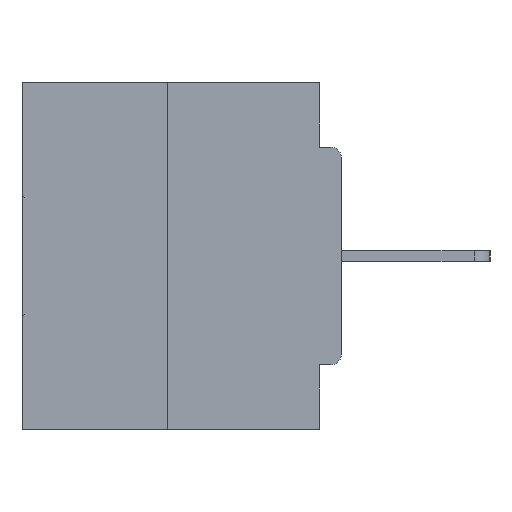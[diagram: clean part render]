
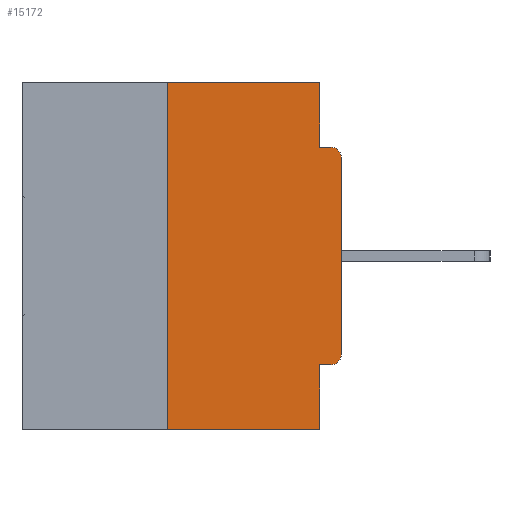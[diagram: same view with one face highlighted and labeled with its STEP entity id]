
A CAD part, left-side view. The second image highlights one B-rep face of the part: STEP entity #15172.
In plain terms, the highlighted planar face has unit normal (-1, 0, 0).
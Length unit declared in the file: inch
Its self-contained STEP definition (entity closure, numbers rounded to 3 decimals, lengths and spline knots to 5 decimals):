
#285 = ORIENTED_EDGE ( 'NONE', *, *, #29070, .F. ) ;
#410 = CARTESIAN_POINT ( 'NONE',  ( 0., 0., -0.1085 ) ) ;
#688 = CARTESIAN_POINT ( 'NONE',  ( 0., 0.25, -0.5 ) ) ;
#1033 = EDGE_CURVE ( 'NONE', #34294, #27503, #32344, .T. ) ;
#1077 = ORIENTED_EDGE ( 'NONE', *, *, #14385, .F. ) ;
#1330 = DIRECTION ( 'NONE',  ( 0., 0., -1. ) ) ;
#1719 = EDGE_CURVE ( 'NONE', #29266, #22250, #33570, .T. ) ;
#1813 = FACE_OUTER_BOUND ( 'NONE', #9121, .T. ) ;
#2770 = CARTESIAN_POINT ( 'NONE',  ( 0., 0.25, 0. ) ) ;
#3342 = DIRECTION ( 'NONE',  ( 0., 1., 0. ) ) ;
#4449 = AXIS2_PLACEMENT_3D ( 'NONE', #12134, #6806, #1330 ) ;
#4674 = DIRECTION ( 'NONE',  ( 0., -1., 0. ) ) ;
#5572 = VECTOR ( 'NONE', #19387, 39.37008 ) ;
#6806 = DIRECTION ( 'NONE',  ( -1., 0., 0. ) ) ;
#7591 = ORIENTED_EDGE ( 'NONE', *, *, #1033, .T. ) ;
#7671 = CARTESIAN_POINT ( 'NONE',  ( 0., 0.46, 0. ) ) ;
#7896 = CARTESIAN_POINT ( 'NONE',  ( 0., 0.015, -0.0935 ) ) ;
#8212 = LINE ( 'NONE', #17017, #31255 ) ;
#9121 = EDGE_LOOP ( 'NONE', ( #16696, #1077, #13691, #285, #24220, #7591, #22147, #12016, #12784, #18666 ) ) ;
#9130 = CARTESIAN_POINT ( 'NONE',  ( 0., 0.46, 0. ) ) ;
#9494 = LINE ( 'NONE', #31753, #15277 ) ;
#9628 = CARTESIAN_POINT ( 'NONE',  ( 0., 0.031, -0.5 ) ) ;
#9995 = EDGE_CURVE ( 'NONE', #34294, #20419, #28713, .T. ) ;
#10006 = VECTOR ( 'NONE', #3342, 39.37008 ) ;
#10246 = VERTEX_POINT ( 'NONE', #2770 ) ;
#10512 = CARTESIAN_POINT ( 'NONE',  ( 0., 0.031, -0.0935 ) ) ;
#10579 = CARTESIAN_POINT ( 'NONE',  ( 0., 0.031, 0. ) ) ;
#11364 = VERTEX_POINT ( 'NONE', #9628 ) ;
#11960 = VECTOR ( 'NONE', #4674, 39.37008 ) ;
#12016 = ORIENTED_EDGE ( 'NONE', *, *, #32471, .T. ) ;
#12068 = CARTESIAN_POINT ( 'NONE',  ( 0., 0.015, -0.3915 ) ) ;
#12134 = CARTESIAN_POINT ( 'NONE',  ( 0., 0.015, -0.1085 ) ) ;
#12256 = LINE ( 'NONE', #34728, #26589 ) ;
#12784 = ORIENTED_EDGE ( 'NONE', *, *, #13802, .F. ) ;
#13243 = LINE ( 'NONE', #35322, #24925 ) ;
#13640 = LINE ( 'NONE', #22123, #14757 ) ;
#13691 = ORIENTED_EDGE ( 'NONE', *, *, #24667, .T. ) ;
#13802 = EDGE_CURVE ( 'NONE', #22250, #20015, #12256, .T. ) ;
#13872 = CARTESIAN_POINT ( 'NONE',  ( 0., 0.031, 0. ) ) ;
#14203 = AXIS2_PLACEMENT_3D ( 'NONE', #7671, #15938, #15387 ) ;
#14385 = EDGE_CURVE ( 'NONE', #26643, #10246, #13640, .T. ) ;
#14757 = VECTOR ( 'NONE', #24898, 39.37008 ) ;
#15002 = DIRECTION ( 'NONE',  ( 0., -1., 0. ) ) ;
#15172 = ADVANCED_FACE ( 'NONE', ( #1813 ), #15579, .F. ) ;
#15277 = VECTOR ( 'NONE', #15002, 39.37008 ) ;
#15280 = EDGE_CURVE ( 'NONE', #27503, #33959, #8212, .T. ) ;
#15387 = DIRECTION ( 'NONE',  ( 0., 0., -1. ) ) ;
#15579 = PLANE ( 'NONE',  #14203 ) ;
#15938 = DIRECTION ( 'NONE',  ( 1., 0., 0. ) ) ;
#16317 = DIRECTION ( 'NONE',  ( 0., 0., 1. ) ) ;
#16696 = ORIENTED_EDGE ( 'NONE', *, *, #16737, .F. ) ;
#16737 = EDGE_CURVE ( 'NONE', #10246, #29266, #34343, .T. ) ;
#17017 = CARTESIAN_POINT ( 'NONE',  ( 0., 0., 0. ) ) ;
#17055 = CARTESIAN_POINT ( 'NONE',  ( 0., 0.015, -0.4065 ) ) ;
#17063 = CARTESIAN_POINT ( 'NONE',  ( 0., 0., -0.3915 ) ) ;
#18666 = ORIENTED_EDGE ( 'NONE', *, *, #1719, .F. ) ;
#19387 = DIRECTION ( 'NONE',  ( 0., 0., -1. ) ) ;
#20015 = VERTEX_POINT ( 'NONE', #7896 ) ;
#20419 = VERTEX_POINT ( 'NONE', #30483 ) ;
#22123 = CARTESIAN_POINT ( 'NONE',  ( 0., 0.25, 0. ) ) ;
#22147 = ORIENTED_EDGE ( 'NONE', *, *, #15280, .T. ) ;
#22250 = VERTEX_POINT ( 'NONE', #10512 ) ;
#23317 = DIRECTION ( 'NONE',  ( -1., 0., 0. ) ) ;
#23332 = DIRECTION ( 'NONE',  ( 0., -1., 0. ) ) ;
#24109 = DIRECTION ( 'NONE',  ( 0., 0., -1. ) ) ;
#24220 = ORIENTED_EDGE ( 'NONE', *, *, #9995, .F. ) ;
#24230 = DIRECTION ( 'NONE',  ( 0., 0., -1. ) ) ;
#24667 = EDGE_CURVE ( 'NONE', #26643, #11364, #9494, .T. ) ;
#24898 = DIRECTION ( 'NONE',  ( 0., 0., 1. ) ) ;
#24925 = VECTOR ( 'NONE', #24109, 39.37008 ) ;
#26589 = VECTOR ( 'NONE', #23332, 39.37008 ) ;
#26643 = VERTEX_POINT ( 'NONE', #688 ) ;
#27503 = VERTEX_POINT ( 'NONE', #17063 ) ;
#28713 = LINE ( 'NONE', #31833, #10006 ) ;
#29070 = EDGE_CURVE ( 'NONE', #20419, #11364, #13243, .T. ) ;
#29266 = VERTEX_POINT ( 'NONE', #10579 ) ;
#30483 = CARTESIAN_POINT ( 'NONE',  ( 0., 0.031, -0.4065 ) ) ;
#30608 = AXIS2_PLACEMENT_3D ( 'NONE', #12068, #23317, #24230 ) ;
#31255 = VECTOR ( 'NONE', #16317, 39.37008 ) ;
#31753 = CARTESIAN_POINT ( 'NONE',  ( 0., 0.46, -0.5 ) ) ;
#31833 = CARTESIAN_POINT ( 'NONE',  ( 0., 0., -0.4065 ) ) ;
#32344 = CIRCLE ( 'NONE', #30608, 0.015 ) ;
#32471 = EDGE_CURVE ( 'NONE', #33959, #20015, #35013, .T. ) ;
#33570 = LINE ( 'NONE', #13872, #5572 ) ;
#33959 = VERTEX_POINT ( 'NONE', #410 ) ;
#34294 = VERTEX_POINT ( 'NONE', #17055 ) ;
#34343 = LINE ( 'NONE', #9130, #11960 ) ;
#34728 = CARTESIAN_POINT ( 'NONE',  ( 0., 0., -0.0935 ) ) ;
#35013 = CIRCLE ( 'NONE', #4449, 0.015 ) ;
#35322 = CARTESIAN_POINT ( 'NONE',  ( 0., 0.031, -0.5 ) ) ;
